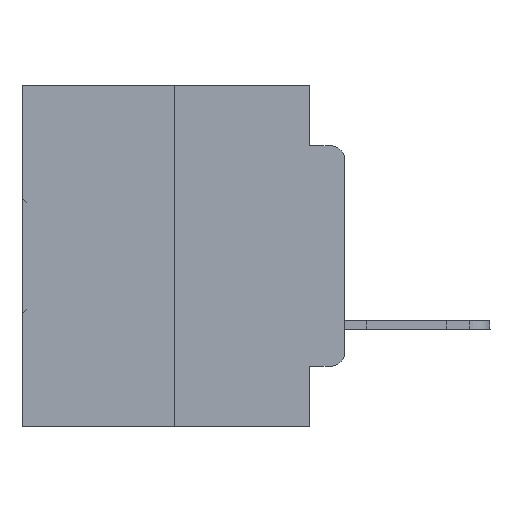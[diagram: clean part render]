
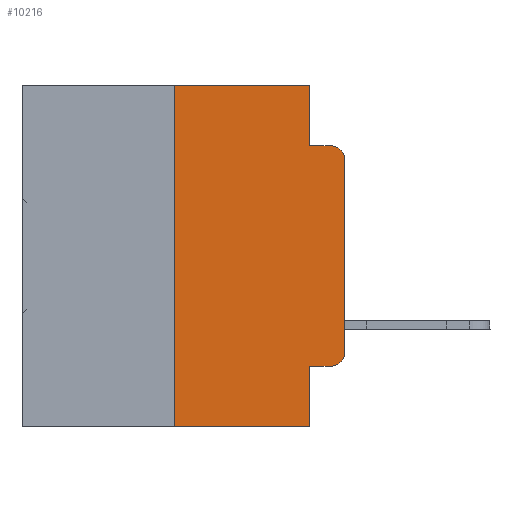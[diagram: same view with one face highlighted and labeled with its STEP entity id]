
A CAD part, left-side view. The second image highlights one B-rep face of the part: STEP entity #10216.
In plain terms, the highlighted planar face has unit normal (-1, 0, 0).
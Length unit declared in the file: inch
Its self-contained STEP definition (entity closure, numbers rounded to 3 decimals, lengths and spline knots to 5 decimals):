
#268 = ORIENTED_EDGE ( 'NONE', *, *, #26688, .F. ) ;
#440 = CARTESIAN_POINT ( 'NONE',  ( 0., 0.02, -0.4115 ) ) ;
#779 = DIRECTION ( 'NONE',  ( 0., 0., 1. ) ) ;
#893 = EDGE_CURVE ( 'NONE', #24726, #26951, #21176, .T. ) ;
#1701 = AXIS2_PLACEMENT_3D ( 'NONE', #25075, #17120, #9020 ) ;
#3522 = VERTEX_POINT ( 'NONE', #16196 ) ;
#3791 = CARTESIAN_POINT ( 'NONE',  ( 0., 0.051, 0. ) ) ;
#4693 = PLANE ( 'NONE',  #31473 ) ;
#4882 = CARTESIAN_POINT ( 'NONE',  ( 0., 0.051, -0.0885 ) ) ;
#4911 = CARTESIAN_POINT ( 'NONE',  ( 0., 0.473, 0. ) ) ;
#5266 = FACE_OUTER_BOUND ( 'NONE', #29338, .T. ) ;
#5651 = CARTESIAN_POINT ( 'NONE',  ( 0., 0., 0. ) ) ;
#5862 = CARTESIAN_POINT ( 'NONE',  ( 0., 0.473, 0. ) ) ;
#6538 = CIRCLE ( 'NONE', #1701, 0.02 ) ;
#7499 = ORIENTED_EDGE ( 'NONE', *, *, #9792, .T. ) ;
#8492 = EDGE_CURVE ( 'NONE', #24793, #24726, #29468, .T. ) ;
#8595 = ORIENTED_EDGE ( 'NONE', *, *, #28537, .T. ) ;
#8718 = ORIENTED_EDGE ( 'NONE', *, *, #893, .F. ) ;
#9020 = DIRECTION ( 'NONE',  ( 0., 0., -1. ) ) ;
#9486 = CARTESIAN_POINT ( 'NONE',  ( 0., 0.051, 0. ) ) ;
#9717 = VERTEX_POINT ( 'NONE', #22147 ) ;
#9792 = EDGE_CURVE ( 'NONE', #11588, #19987, #6538, .T. ) ;
#10099 = ORIENTED_EDGE ( 'NONE', *, *, #31041, .T. ) ;
#10100 = LINE ( 'NONE', #9486, #29236 ) ;
#10216 = ADVANCED_FACE ( 'NONE', ( #5266 ), #4693, .F. ) ;
#10711 = DIRECTION ( 'NONE',  ( 0., 0., 1. ) ) ;
#11410 = CARTESIAN_POINT ( 'NONE',  ( 0., 0.02, -0.3915 ) ) ;
#11588 = VERTEX_POINT ( 'NONE', #24084 ) ;
#13785 = VECTOR ( 'NONE', #19265, 39.37008 ) ;
#14050 = DIRECTION ( 'NONE',  ( 0., 0., -1. ) ) ;
#14740 = DIRECTION ( 'NONE',  ( 0., 0., -1. ) ) ;
#16196 = CARTESIAN_POINT ( 'NONE',  ( 0., 0.051, -0.5 ) ) ;
#16210 = LINE ( 'NONE', #5651, #16632 ) ;
#16326 = DIRECTION ( 'NONE',  ( 0., -1., 0. ) ) ;
#16632 = VECTOR ( 'NONE', #10711, 39.37008 ) ;
#17120 = DIRECTION ( 'NONE',  ( -1., 0., 0. ) ) ;
#18891 = VECTOR ( 'NONE', #32109, 39.37008 ) ;
#19265 = DIRECTION ( 'NONE',  ( 0., -1., 0. ) ) ;
#19619 = VECTOR ( 'NONE', #16326, 39.37008 ) ;
#19874 = AXIS2_PLACEMENT_3D ( 'NONE', #11410, #32155, #14050 ) ;
#19911 = CARTESIAN_POINT ( 'NONE',  ( 0., 0.051, -0.4115 ) ) ;
#19987 = VERTEX_POINT ( 'NONE', #21071 ) ;
#20542 = CARTESIAN_POINT ( 'NONE',  ( 0., 0., -0.3915 ) ) ;
#20745 = CARTESIAN_POINT ( 'NONE',  ( 0., 0.051, 0. ) ) ;
#21071 = CARTESIAN_POINT ( 'NONE',  ( 0., 0.02, -0.0885 ) ) ;
#21176 = LINE ( 'NONE', #20745, #26050 ) ;
#21636 = CARTESIAN_POINT ( 'NONE',  ( 0., 0.25, 0. ) ) ;
#22147 = CARTESIAN_POINT ( 'NONE',  ( 0., 0.25, -0.5 ) ) ;
#22439 = CARTESIAN_POINT ( 'NONE',  ( 0., 0.25, 0. ) ) ;
#22813 = EDGE_CURVE ( 'NONE', #9717, #3522, #25730, .T. ) ;
#23062 = VECTOR ( 'NONE', #31465, 39.37008 ) ;
#23176 = LINE ( 'NONE', #25059, #13785 ) ;
#23196 = DIRECTION ( 'NONE',  ( 1., 0., 0. ) ) ;
#23547 = DIRECTION ( 'NONE',  ( 0., 0., -1. ) ) ;
#24084 = CARTESIAN_POINT ( 'NONE',  ( 0., 0., -0.1085 ) ) ;
#24726 = VERTEX_POINT ( 'NONE', #3791 ) ;
#24793 = VERTEX_POINT ( 'NONE', #22439 ) ;
#25059 = CARTESIAN_POINT ( 'NONE',  ( 0., 0.051, -0.4115 ) ) ;
#25060 = CARTESIAN_POINT ( 'NONE',  ( 0., 0.051, -0.0885 ) ) ;
#25075 = CARTESIAN_POINT ( 'NONE',  ( 0., 0.02, -0.1085 ) ) ;
#25104 = VERTEX_POINT ( 'NONE', #440 ) ;
#25480 = VERTEX_POINT ( 'NONE', #19911 ) ;
#25510 = LINE ( 'NONE', #4882, #23062 ) ;
#25730 = LINE ( 'NONE', #29521, #19619 ) ;
#26050 = VECTOR ( 'NONE', #23547, 39.37008 ) ;
#26491 = VECTOR ( 'NONE', #779, 39.37008 ) ;
#26688 = EDGE_CURVE ( 'NONE', #26951, #19987, #25510, .T. ) ;
#26908 = ORIENTED_EDGE ( 'NONE', *, *, #30539, .T. ) ;
#26951 = VERTEX_POINT ( 'NONE', #25060 ) ;
#27009 = ORIENTED_EDGE ( 'NONE', *, *, #28686, .F. ) ;
#27190 = ORIENTED_EDGE ( 'NONE', *, *, #27837, .F. ) ;
#27837 = EDGE_CURVE ( 'NONE', #9717, #24793, #30166, .T. ) ;
#28537 = EDGE_CURVE ( 'NONE', #25104, #33835, #30071, .T. ) ;
#28613 = ORIENTED_EDGE ( 'NONE', *, *, #8492, .F. ) ;
#28686 = EDGE_CURVE ( 'NONE', #25480, #3522, #10100, .T. ) ;
#29236 = VECTOR ( 'NONE', #14740, 39.37008 ) ;
#29338 = EDGE_LOOP ( 'NONE', ( #10099, #7499, #268, #8718, #28613, #27190, #30784, #27009, #26908, #8595 ) ) ;
#29468 = LINE ( 'NONE', #5862, #18891 ) ;
#29521 = CARTESIAN_POINT ( 'NONE',  ( 0., 0.473, -0.5 ) ) ;
#30071 = CIRCLE ( 'NONE', #19874, 0.02 ) ;
#30166 = LINE ( 'NONE', #21636, #26491 ) ;
#30539 = EDGE_CURVE ( 'NONE', #25480, #25104, #23176, .T. ) ;
#30784 = ORIENTED_EDGE ( 'NONE', *, *, #22813, .T. ) ;
#31041 = EDGE_CURVE ( 'NONE', #33835, #11588, #16210, .T. ) ;
#31465 = DIRECTION ( 'NONE',  ( 0., -1., 0. ) ) ;
#31473 = AXIS2_PLACEMENT_3D ( 'NONE', #4911, #23196, #33681 ) ;
#32109 = DIRECTION ( 'NONE',  ( 0., -1., 0. ) ) ;
#32155 = DIRECTION ( 'NONE',  ( -1., 0., 0. ) ) ;
#33681 = DIRECTION ( 'NONE',  ( 0., 0., -1. ) ) ;
#33835 = VERTEX_POINT ( 'NONE', #20542 ) ;
